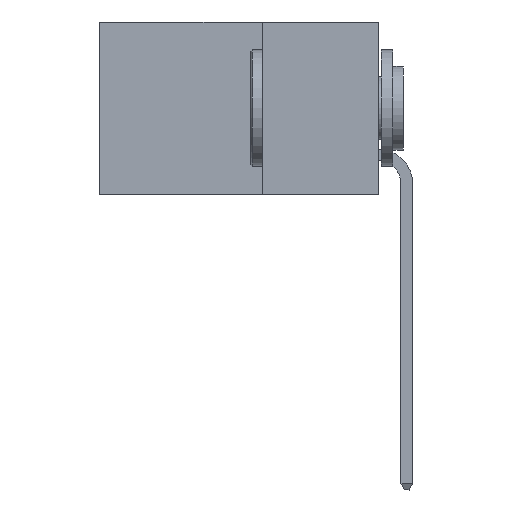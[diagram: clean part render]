
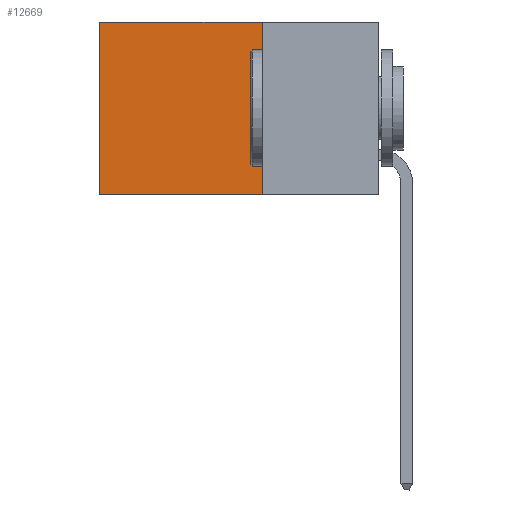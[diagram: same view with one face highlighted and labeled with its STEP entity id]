
A CAD part, left-side view. The second image highlights one B-rep face of the part: STEP entity #12669.
In plain terms, the highlighted planar face has unit normal (-1, 0, 0).
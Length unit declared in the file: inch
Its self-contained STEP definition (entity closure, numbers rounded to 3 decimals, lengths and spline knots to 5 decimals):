
#64 = ORIENTED_EDGE ( 'NONE', *, *, #7259, .F. ) ;
#382 = CARTESIAN_POINT ( 'NONE',  ( 0.298, 0.25, 0. ) ) ;
#548 = VERTEX_POINT ( 'NONE', #9180 ) ;
#573 = PLANE ( 'NONE',  #6172 ) ;
#3519 = CARTESIAN_POINT ( 'NONE',  ( 0.298, 0.25, -0.37 ) ) ;
#4064 = LINE ( 'NONE', #24174, #17753 ) ;
#5087 = ORIENTED_EDGE ( 'NONE', *, *, #14591, .F. ) ;
#6000 = CARTESIAN_POINT ( 'NONE',  ( 0.298, 0.25, 0. ) ) ;
#6172 = AXIS2_PLACEMENT_3D ( 'NONE', #382, #24868, #10607 ) ;
#7180 = DIRECTION ( 'NONE',  ( 0., 0., -1. ) ) ;
#7259 = EDGE_CURVE ( 'NONE', #17671, #548, #24585, .T. ) ;
#7430 = CARTESIAN_POINT ( 'NONE',  ( 0.298, 0.25, 0. ) ) ;
#7711 = EDGE_LOOP ( 'NONE', ( #11514, #5087, #64, #19306 ) ) ;
#8209 = CARTESIAN_POINT ( 'NONE',  ( 0.298, 0.25, 0. ) ) ;
#9033 = FACE_OUTER_BOUND ( 'NONE', #7711, .T. ) ;
#9180 = CARTESIAN_POINT ( 'NONE',  ( 0.298, 0.25, -0.37 ) ) ;
#10607 = DIRECTION ( 'NONE',  ( 0., 0., -1. ) ) ;
#11514 = ORIENTED_EDGE ( 'NONE', *, *, #13599, .T. ) ;
#12669 = ADVANCED_FACE ( 'NONE', ( #9033 ), #573, .F. ) ;
#13055 = EDGE_CURVE ( 'NONE', #17671, #13685, #23007, .T. ) ;
#13599 = EDGE_CURVE ( 'NONE', #13685, #18985, #4064, .T. ) ;
#13685 = VERTEX_POINT ( 'NONE', #20513 ) ;
#14037 = DIRECTION ( 'NONE',  ( 0., 0., -1. ) ) ;
#14591 = EDGE_CURVE ( 'NONE', #548, #18985, #23757, .T. ) ;
#16326 = VECTOR ( 'NONE', #18861, 39.37008 ) ;
#17671 = VERTEX_POINT ( 'NONE', #8209 ) ;
#17753 = VECTOR ( 'NONE', #14037, 39.37008 ) ;
#18861 = DIRECTION ( 'NONE',  ( 0., 1., 0. ) ) ;
#18985 = VERTEX_POINT ( 'NONE', #25038 ) ;
#19306 = ORIENTED_EDGE ( 'NONE', *, *, #13055, .T. ) ;
#19817 = DIRECTION ( 'NONE',  ( 0., 1., 0. ) ) ;
#20513 = CARTESIAN_POINT ( 'NONE',  ( 0.298, 0.6, 0. ) ) ;
#21450 = VECTOR ( 'NONE', #7180, 39.37008 ) ;
#23007 = LINE ( 'NONE', #6000, #16326 ) ;
#23757 = LINE ( 'NONE', #3519, #25344 ) ;
#24174 = CARTESIAN_POINT ( 'NONE',  ( 0.298, 0.6, 0. ) ) ;
#24585 = LINE ( 'NONE', #7430, #21450 ) ;
#24868 = DIRECTION ( 'NONE',  ( 1., 0., 0. ) ) ;
#25038 = CARTESIAN_POINT ( 'NONE',  ( 0.298, 0.6, -0.37 ) ) ;
#25344 = VECTOR ( 'NONE', #19817, 39.37008 ) ;
